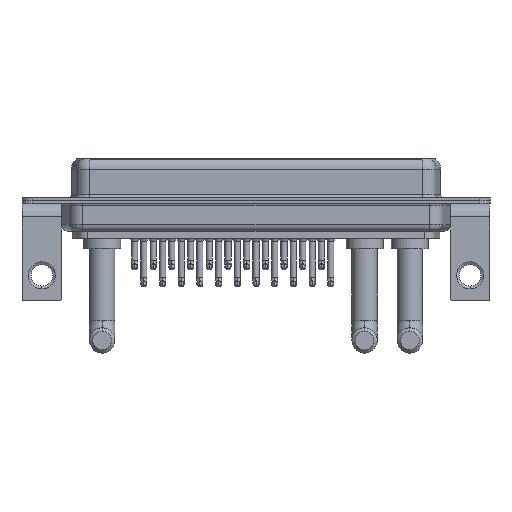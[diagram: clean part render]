
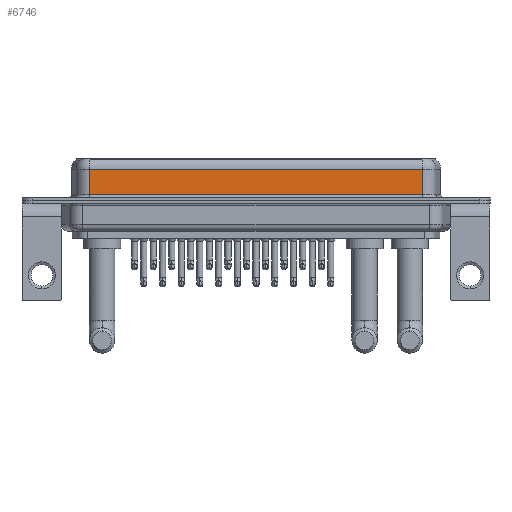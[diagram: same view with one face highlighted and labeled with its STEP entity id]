
A CAD part, front view. The second image highlights one B-rep face of the part: STEP entity #6746.
In plain terms, the highlighted planar face has unit normal (0, -1, 0).
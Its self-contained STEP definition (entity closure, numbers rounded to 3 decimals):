
#182 = EDGE_CURVE ( 'NONE', #7248, #22643, #3598, .T. ) ;
#335 = AXIS2_PLACEMENT_3D ( 'NONE', #14519, #5194, #20258 ) ;
#355 = CARTESIAN_POINT ( 'NONE',  ( 56.462, -3.95, 4.65 ) ) ;
#581 = ORIENTED_EDGE ( 'NONE', *, *, #19802, .T. ) ;
#1263 = CARTESIAN_POINT ( 'NONE',  ( 56.462, -3.95, 0.9 ) ) ;
#1490 = CARTESIAN_POINT ( 'NONE',  ( 56.462, -3.95, 6.4 ) ) ;
#3598 = LINE ( 'NONE', #1490, #13622 ) ;
#4268 = VECTOR ( 'NONE', #7923, 1000. ) ;
#5194 = DIRECTION ( 'NONE',  ( 0., 1., 0. ) ) ;
#6746 = ADVANCED_FACE ( 'NONE', ( #18251 ), #6926, .F. ) ;
#6926 = PLANE ( 'NONE',  #335 ) ;
#7248 = VERTEX_POINT ( 'NONE', #23068 ) ;
#7923 = DIRECTION ( 'NONE',  ( -1., 0., 0. ) ) ;
#8246 = EDGE_CURVE ( 'NONE', #7248, #23661, #15380, .T. ) ;
#9111 = DIRECTION ( 'NONE',  ( 1., 0., 0. ) ) ;
#9405 = ORIENTED_EDGE ( 'NONE', *, *, #182, .F. ) ;
#10213 = ORIENTED_EDGE ( 'NONE', *, *, #15968, .T. ) ;
#11191 = DIRECTION ( 'NONE',  ( 0., 0., -1. ) ) ;
#11297 = DIRECTION ( 'NONE',  ( 0., 0., -1. ) ) ;
#12982 = ORIENTED_EDGE ( 'NONE', *, *, #8246, .T. ) ;
#13039 = CARTESIAN_POINT ( 'NONE',  ( 7.038, -3.95, 6.4 ) ) ;
#13218 = LINE ( 'NONE', #24281, #23595 ) ;
#13622 = VECTOR ( 'NONE', #11191, 1000. ) ;
#14519 = CARTESIAN_POINT ( 'NONE',  ( 56.462, -3.95, 6.4 ) ) ;
#15272 = CARTESIAN_POINT ( 'NONE',  ( 7.038, -3.95, 0.9 ) ) ;
#15380 = LINE ( 'NONE', #355, #4268 ) ;
#15968 = EDGE_CURVE ( 'NONE', #20004, #22643, #13218, .T. ) ;
#18251 = FACE_OUTER_BOUND ( 'NONE', #21654, .T. ) ;
#19802 = EDGE_CURVE ( 'NONE', #23661, #20004, #22263, .T. ) ;
#20004 = VERTEX_POINT ( 'NONE', #15272 ) ;
#20258 = DIRECTION ( 'NONE',  ( 0., 0., 1. ) ) ;
#21654 = EDGE_LOOP ( 'NONE', ( #9405, #12982, #581, #10213 ) ) ;
#21993 = CARTESIAN_POINT ( 'NONE',  ( 7.038, -3.95, 4.65 ) ) ;
#22263 = LINE ( 'NONE', #13039, #22994 ) ;
#22643 = VERTEX_POINT ( 'NONE', #1263 ) ;
#22994 = VECTOR ( 'NONE', #11297, 1000. ) ;
#23068 = CARTESIAN_POINT ( 'NONE',  ( 56.462, -3.95, 4.65 ) ) ;
#23595 = VECTOR ( 'NONE', #9111, 1000. ) ;
#23661 = VERTEX_POINT ( 'NONE', #21993 ) ;
#24281 = CARTESIAN_POINT ( 'NONE',  ( 56.462, -3.95, 0.9 ) ) ;
